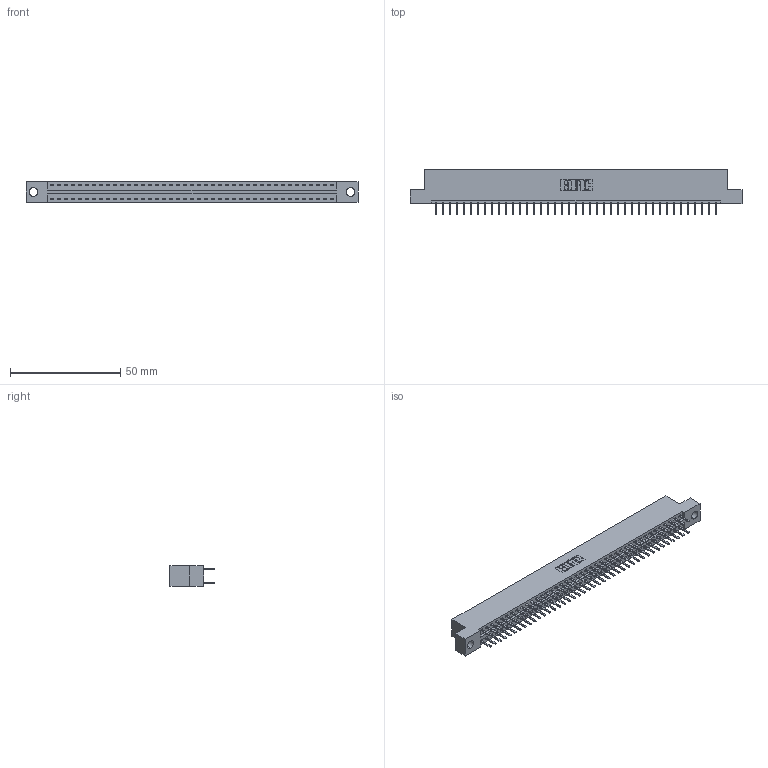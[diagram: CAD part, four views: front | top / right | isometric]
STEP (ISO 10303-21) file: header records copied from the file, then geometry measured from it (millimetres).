
FILE_DESCRIPTION (( 'STEP AP203' ), '1' );
FILE_NAME ('346-082-520-204.STEP', '2022-05-25T17:09:16', ( '' ), ( '' ), 'SwSTEP 2.0', 'SolidWorks 2020', '' );
FILE_SCHEMA (( 'CONFIG_CONTROL_DESIGN' ));
Length unit declared in the file: inch
Products named in the file (3): 346-082-520-204; 345-292-001_345-293-120; 346 Part_Flush Mounting Lugs - 0.156 Dia-TH
Assembly tree (83 placements, depth 2):
  346-082-520-204
    346 Part_Flush Mounting Lugs - 0.156 Dia-TH
    345-292-001_345-293-120  x82
Bounding box: 150.75 x 20.02 x 9.4 mm (x, y, z)
Volume: 14550.1 mm3; surface area: 19747.8 mm2
Topology: 83 solids, 83 shells, 4728 faces, 13731 edges, 8934 vertices
Faces by surface type: plane 3124, cylinder 1604
Entity records: 27425 total; most frequent: CARTESIAN_POINT 4538, ORIENTED_EDGE 4458, DIRECTION 4037, EDGE_CURVE 2229, LINE 1929, VECTOR 1929, VERTEX_POINT 1482, AXIS2_PLACEMENT_3D 1054
